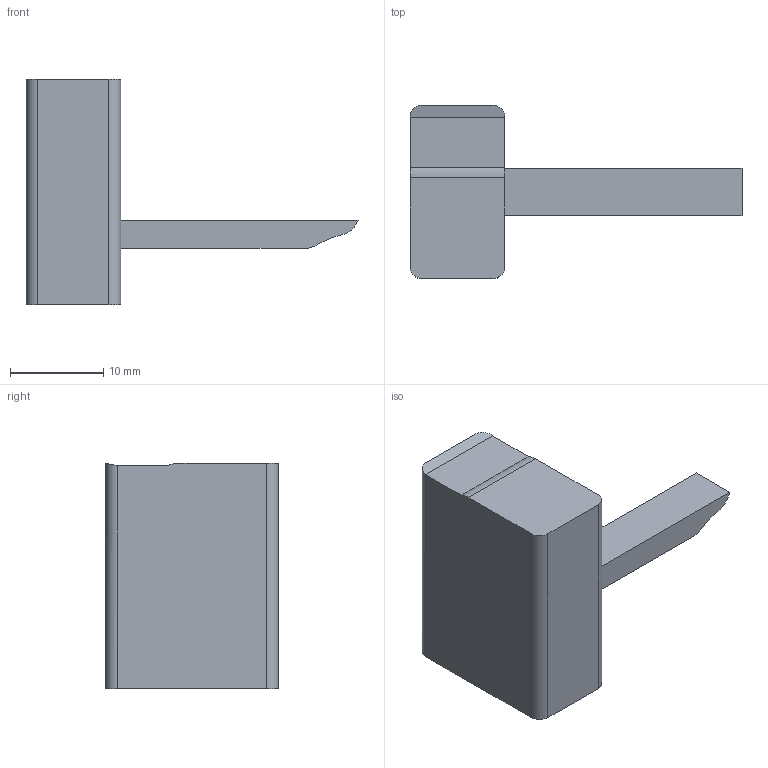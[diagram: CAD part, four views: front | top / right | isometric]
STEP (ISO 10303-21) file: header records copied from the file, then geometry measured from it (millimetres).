
FILE_DESCRIPTION (( 'STEP AP214' ), '1' );
FILE_NAME ('striker.STEP', '2014-01-22T21:34:01', ( '' ), ( '' ), 'SwSTEP 2.0', 'SolidWorks 2013', '' );
FILE_SCHEMA (( 'AUTOMOTIVE_DESIGN' ));
Length unit declared in the file: inch
Products named in the file (1): striker
Bounding box: 35.56 x 18.54 x 24.13 mm (x, y, z)
Volume: 4853.8 mm3; surface area: 2092.6 mm2
Topology: 1 solids, 1 shells, 20 faces, 49 edges, 32 vertices
Faces by surface type: plane 12, cylinder 8
Entity records: 631 total; most frequent: CARTESIAN_POINT 108, DIRECTION 103, ORIENTED_EDGE 98, EDGE_CURVE 49, AXIS2_PLACEMENT_3D 35, LINE 33, VECTOR 33, VERTEX_POINT 32
